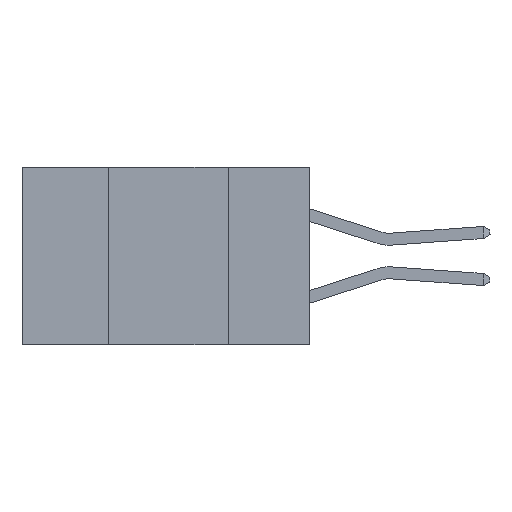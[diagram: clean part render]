
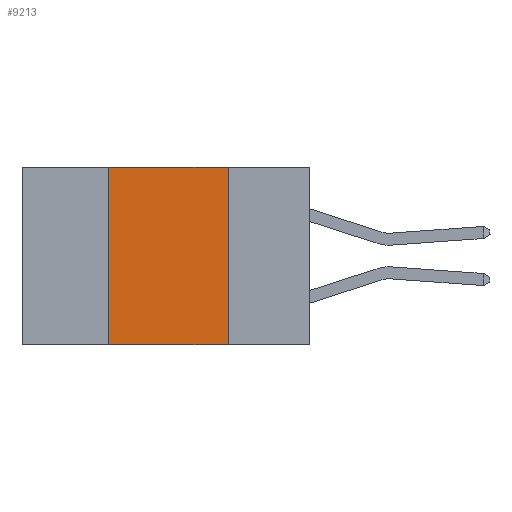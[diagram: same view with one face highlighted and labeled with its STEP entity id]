
A CAD part, left-side view. The second image highlights one B-rep face of the part: STEP entity #9213.
In plain terms, the highlighted planar face has unit normal (-1, 0, 0).
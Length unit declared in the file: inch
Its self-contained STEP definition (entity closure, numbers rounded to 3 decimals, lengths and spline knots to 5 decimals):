
#381 = DIRECTION ( 'NONE',  ( 0., -1., 0. ) ) ;
#567 = CARTESIAN_POINT ( 'NONE',  ( 0., 0.42, 0. ) ) ;
#1019 = VERTEX_POINT ( 'NONE', #2229 ) ;
#1798 = FACE_OUTER_BOUND ( 'NONE', #3009, .T. ) ;
#1882 = VERTEX_POINT ( 'NONE', #9469 ) ;
#2229 = CARTESIAN_POINT ( 'NONE',  ( 0., 0.17, 0. ) ) ;
#2938 = LINE ( 'NONE', #3466, #7791 ) ;
#3009 = EDGE_LOOP ( 'NONE', ( #8877, #7525, #4730, #8228 ) ) ;
#3374 = DIRECTION ( 'NONE',  ( 1., 0., 0. ) ) ;
#3466 = CARTESIAN_POINT ( 'NONE',  ( 0., 0.17, 0. ) ) ;
#3763 = CARTESIAN_POINT ( 'NONE',  ( 0., 0.6, 0. ) ) ;
#3802 = VECTOR ( 'NONE', #5025, 39.37008 ) ;
#3924 = LINE ( 'NONE', #11204, #9728 ) ;
#4203 = EDGE_CURVE ( 'NONE', #5560, #1019, #7145, .T. ) ;
#4730 = ORIENTED_EDGE ( 'NONE', *, *, #4980, .F. ) ;
#4932 = VECTOR ( 'NONE', #381, 39.37008 ) ;
#4980 = EDGE_CURVE ( 'NONE', #5773, #5560, #8512, .T. ) ;
#5025 = DIRECTION ( 'NONE',  ( 0., 0., 1. ) ) ;
#5040 = CARTESIAN_POINT ( 'NONE',  ( 0., 0.6, 0. ) ) ;
#5560 = VERTEX_POINT ( 'NONE', #9453 ) ;
#5641 = EDGE_CURVE ( 'NONE', #5773, #1882, #3924, .T. ) ;
#5773 = VERTEX_POINT ( 'NONE', #6024 ) ;
#6024 = CARTESIAN_POINT ( 'NONE',  ( 0., 0.42, -0.37 ) ) ;
#7145 = LINE ( 'NONE', #3763, #4932 ) ;
#7354 = EDGE_CURVE ( 'NONE', #1019, #1882, #2938, .T. ) ;
#7525 = ORIENTED_EDGE ( 'NONE', *, *, #4203, .F. ) ;
#7791 = VECTOR ( 'NONE', #11370, 39.37008 ) ;
#7821 = PLANE ( 'NONE',  #8109 ) ;
#8109 = AXIS2_PLACEMENT_3D ( 'NONE', #5040, #3374, #11305 ) ;
#8228 = ORIENTED_EDGE ( 'NONE', *, *, #5641, .T. ) ;
#8512 = LINE ( 'NONE', #567, #3802 ) ;
#8877 = ORIENTED_EDGE ( 'NONE', *, *, #7354, .F. ) ;
#9213 = ADVANCED_FACE ( 'NONE', ( #1798 ), #7821, .F. ) ;
#9453 = CARTESIAN_POINT ( 'NONE',  ( 0., 0.42, 0. ) ) ;
#9469 = CARTESIAN_POINT ( 'NONE',  ( 0., 0.17, -0.37 ) ) ;
#9728 = VECTOR ( 'NONE', #11130, 39.37008 ) ;
#11130 = DIRECTION ( 'NONE',  ( 0., -1., 0. ) ) ;
#11204 = CARTESIAN_POINT ( 'NONE',  ( 0., 0.6, -0.37 ) ) ;
#11305 = DIRECTION ( 'NONE',  ( 0., 0., -1. ) ) ;
#11370 = DIRECTION ( 'NONE',  ( 0., 0., -1. ) ) ;
